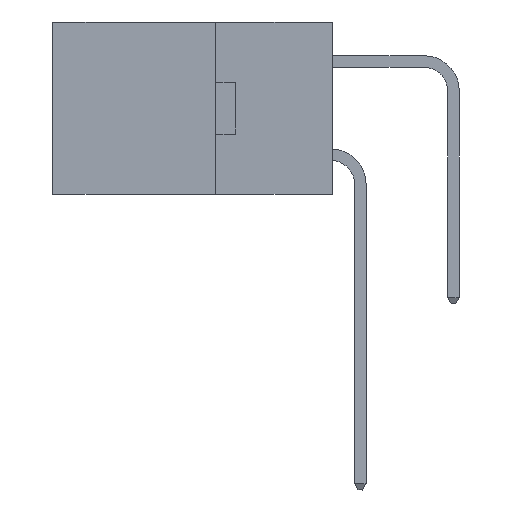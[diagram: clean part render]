
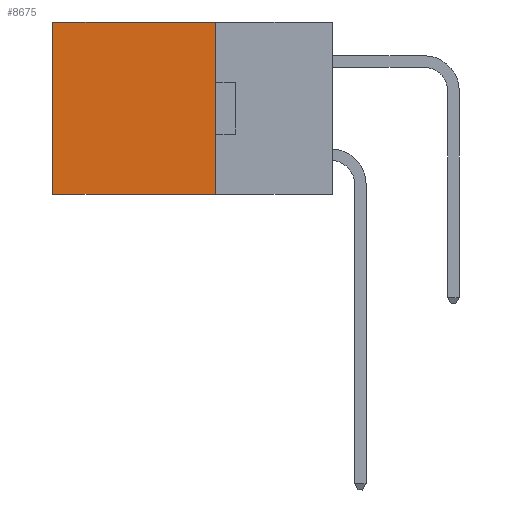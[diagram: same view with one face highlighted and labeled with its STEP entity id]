
A CAD part, left-side view. The second image highlights one B-rep face of the part: STEP entity #8675.
In plain terms, the highlighted planar face has unit normal (-1, 0, 0).
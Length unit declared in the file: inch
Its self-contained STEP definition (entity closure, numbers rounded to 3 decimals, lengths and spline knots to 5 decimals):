
#555 = CARTESIAN_POINT ( 'NONE',  ( 0.2615, 0.25, 0. ) ) ;
#1049 = VERTEX_POINT ( 'NONE', #7246 ) ;
#1120 = ORIENTED_EDGE ( 'NONE', *, *, #14468, .T. ) ;
#1462 = VECTOR ( 'NONE', #5047, 39.37008 ) ;
#2508 = LINE ( 'NONE', #7598, #23326 ) ;
#5047 = DIRECTION ( 'NONE',  ( 0., 1., 0. ) ) ;
#7131 = EDGE_CURVE ( 'NONE', #14806, #12036, #14693, .T. ) ;
#7246 = CARTESIAN_POINT ( 'NONE',  ( 0.2615, 0.25, 0. ) ) ;
#7360 = LINE ( 'NONE', #555, #1462 ) ;
#7572 = DIRECTION ( 'NONE',  ( 0., 1., 0. ) ) ;
#7598 = CARTESIAN_POINT ( 'NONE',  ( 0.2615, 0.25, -0.37 ) ) ;
#8106 = EDGE_LOOP ( 'NONE', ( #21026, #29139, #18002, #1120 ) ) ;
#8675 = ADVANCED_FACE ( 'NONE', ( #13902 ), #13012, .F. ) ;
#9338 = CARTESIAN_POINT ( 'NONE',  ( 0.2615, 0.25, -0.37 ) ) ;
#10119 = EDGE_CURVE ( 'NONE', #26096, #12036, #24741, .T. ) ;
#10547 = CARTESIAN_POINT ( 'NONE',  ( 0.2615, 0.25, -0.37 ) ) ;
#10853 = DIRECTION ( 'NONE',  ( 1., 0., 0. ) ) ;
#12036 = VERTEX_POINT ( 'NONE', #23151 ) ;
#13012 = PLANE ( 'NONE',  #18124 ) ;
#13114 = CARTESIAN_POINT ( 'NONE',  ( 0.2615, 0.6, -0.37 ) ) ;
#13902 = FACE_OUTER_BOUND ( 'NONE', #8106, .T. ) ;
#14468 = EDGE_CURVE ( 'NONE', #1049, #26096, #7360, .T. ) ;
#14693 = LINE ( 'NONE', #28775, #21534 ) ;
#14806 = VERTEX_POINT ( 'NONE', #9338 ) ;
#16864 = EDGE_CURVE ( 'NONE', #1049, #14806, #2508, .T. ) ;
#18002 = ORIENTED_EDGE ( 'NONE', *, *, #16864, .F. ) ;
#18124 = AXIS2_PLACEMENT_3D ( 'NONE', #10547, #10853, #19993 ) ;
#19993 = DIRECTION ( 'NONE',  ( 0., 0., -1. ) ) ;
#21026 = ORIENTED_EDGE ( 'NONE', *, *, #10119, .T. ) ;
#21534 = VECTOR ( 'NONE', #7572, 39.37008 ) ;
#22576 = DIRECTION ( 'NONE',  ( 0., 0., -1. ) ) ;
#23151 = CARTESIAN_POINT ( 'NONE',  ( 0.2615, 0.6, -0.37 ) ) ;
#23326 = VECTOR ( 'NONE', #28511, 39.37008 ) ;
#24741 = LINE ( 'NONE', #13114, #30035 ) ;
#25937 = CARTESIAN_POINT ( 'NONE',  ( 0.2615, 0.6, 0. ) ) ;
#26096 = VERTEX_POINT ( 'NONE', #25937 ) ;
#28511 = DIRECTION ( 'NONE',  ( 0., 0., -1. ) ) ;
#28775 = CARTESIAN_POINT ( 'NONE',  ( 0.2615, 0.25, -0.37 ) ) ;
#29139 = ORIENTED_EDGE ( 'NONE', *, *, #7131, .F. ) ;
#30035 = VECTOR ( 'NONE', #22576, 39.37008 ) ;
